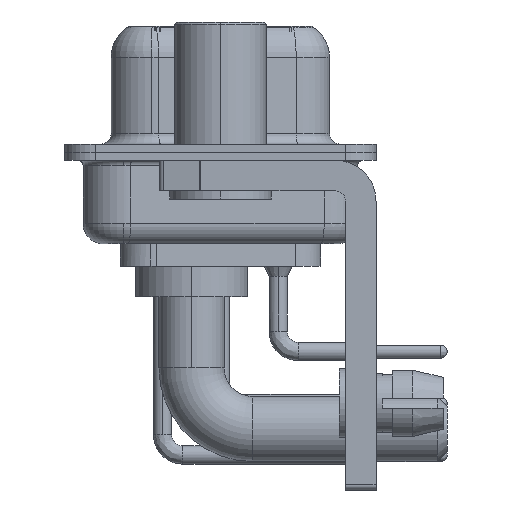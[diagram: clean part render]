
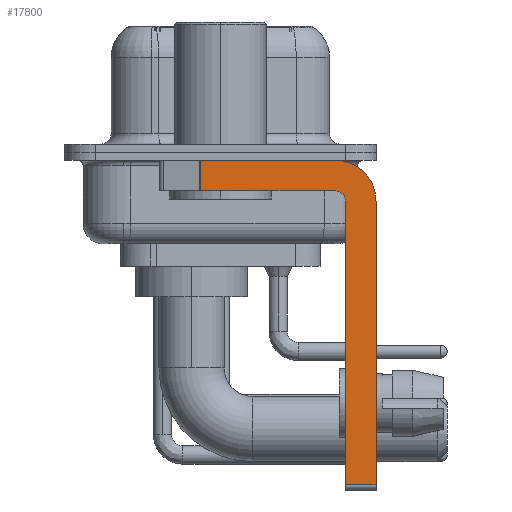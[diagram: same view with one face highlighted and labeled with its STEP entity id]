
A CAD part, left-side view. The second image highlights one B-rep face of the part: STEP entity #17800.
In plain terms, the highlighted planar face has unit normal (-1, 0, 0).
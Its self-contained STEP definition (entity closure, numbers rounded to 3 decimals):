
#389 = VERTEX_POINT ( 'NONE', #1475 ) ;
#677 = AXIS2_PLACEMENT_3D ( 'NONE', #33064, #6649, #15701 ) ;
#1475 = CARTESIAN_POINT ( 'NONE',  ( -2.9, 0.978, -1.9 ) ) ;
#1674 = LINE ( 'NONE', #5129, #32467 ) ;
#1938 = LINE ( 'NONE', #31788, #30900 ) ;
#2028 = LINE ( 'NONE', #25527, #17283 ) ;
#2201 = ORIENTED_EDGE ( 'NONE', *, *, #25031, .T. ) ;
#3866 = CARTESIAN_POINT ( 'NONE',  ( -2.9, -7.65, -2.4 ) ) ;
#3935 = AXIS2_PLACEMENT_3D ( 'NONE', #27962, #4063, #18531 ) ;
#4063 = DIRECTION ( 'NONE',  ( 1., 0., 0. ) ) ;
#4887 = VERTEX_POINT ( 'NONE', #8869 ) ;
#5129 = CARTESIAN_POINT ( 'NONE',  ( -2.9, 3., -0.4 ) ) ;
#5959 = LINE ( 'NONE', #26397, #6907 ) ;
#6649 = DIRECTION ( 'NONE',  ( -1., 0., 0. ) ) ;
#6763 = FACE_OUTER_BOUND ( 'NONE', #11766, .T. ) ;
#6823 = CIRCLE ( 'NONE', #677, 0.5 ) ;
#6907 = VECTOR ( 'NONE', #32362, 1000. ) ;
#7520 = PLANE ( 'NONE',  #3935 ) ;
#8081 = DIRECTION ( 'NONE',  ( 0., 0., 1. ) ) ;
#8353 = ORIENTED_EDGE ( 'NONE', *, *, #16531, .F. ) ;
#8869 = CARTESIAN_POINT ( 'NONE',  ( -2.9, -6.15, -16.35 ) ) ;
#9075 = VECTOR ( 'NONE', #13541, 1000. ) ;
#10257 = VERTEX_POINT ( 'NONE', #33871 ) ;
#10766 = VERTEX_POINT ( 'NONE', #16706 ) ;
#11649 = CIRCLE ( 'NONE', #35049, 2. ) ;
#11766 = EDGE_LOOP ( 'NONE', ( #28055, #37868, #34903, #28811, #8353, #2201, #26903, #27491 ) ) ;
#12780 = CARTESIAN_POINT ( 'NONE',  ( -2.9, -5.65, -16.35 ) ) ;
#13541 = DIRECTION ( 'NONE',  ( 0., -1., 0. ) ) ;
#13992 = CARTESIAN_POINT ( 'NONE',  ( -2.9, -5.65, -1.9 ) ) ;
#15282 = LINE ( 'NONE', #29932, #34259 ) ;
#15701 = DIRECTION ( 'NONE',  ( 0., 0., 1. ) ) ;
#16531 = EDGE_CURVE ( 'NONE', #4887, #10257, #1938, .T. ) ;
#16626 = EDGE_CURVE ( 'NONE', #31880, #10766, #5959, .T. ) ;
#16664 = DIRECTION ( 'NONE',  ( 0., 1., 0. ) ) ;
#16706 = CARTESIAN_POINT ( 'NONE',  ( -2.9, -7.65, -16.35 ) ) ;
#16936 = CARTESIAN_POINT ( 'NONE',  ( -2.9, 0.978, -0.4 ) ) ;
#17283 = VECTOR ( 'NONE', #16664, 1000. ) ;
#17800 = ADVANCED_FACE ( 'NONE', ( #6763 ), #7520, .F. ) ;
#18531 = DIRECTION ( 'NONE',  ( 0., 0., -1. ) ) ;
#18660 = DIRECTION ( 'NONE',  ( 1., 0., 0. ) ) ;
#18956 = LINE ( 'NONE', #12780, #9075 ) ;
#19241 = VERTEX_POINT ( 'NONE', #32858 ) ;
#21357 = DIRECTION ( 'NONE',  ( 0., 0., -1. ) ) ;
#24742 = DIRECTION ( 'NONE',  ( 0., 0., -1. ) ) ;
#25031 = EDGE_CURVE ( 'NONE', #4887, #10766, #18956, .T. ) ;
#25527 = CARTESIAN_POINT ( 'NONE',  ( -2.9, -5.65, -1.9 ) ) ;
#26397 = CARTESIAN_POINT ( 'NONE',  ( -2.9, -7.65, -2.4 ) ) ;
#26903 = ORIENTED_EDGE ( 'NONE', *, *, #16626, .F. ) ;
#27491 = ORIENTED_EDGE ( 'NONE', *, *, #37072, .F. ) ;
#27936 = EDGE_CURVE ( 'NONE', #10257, #32421, #6823, .T. ) ;
#27962 = CARTESIAN_POINT ( 'NONE',  ( -2.9, -5.65, -2.4 ) ) ;
#28055 = ORIENTED_EDGE ( 'NONE', *, *, #34947, .F. ) ;
#28811 = ORIENTED_EDGE ( 'NONE', *, *, #27936, .F. ) ;
#29322 = EDGE_CURVE ( 'NONE', #32421, #389, #2028, .T. ) ;
#29932 = CARTESIAN_POINT ( 'NONE',  ( -2.9, 0.978, -1.9 ) ) ;
#30900 = VECTOR ( 'NONE', #8081, 1000. ) ;
#31788 = CARTESIAN_POINT ( 'NONE',  ( -2.9, -6.15, -16.6 ) ) ;
#31880 = VERTEX_POINT ( 'NONE', #3866 ) ;
#32362 = DIRECTION ( 'NONE',  ( 0., 0., -1. ) ) ;
#32421 = VERTEX_POINT ( 'NONE', #13992 ) ;
#32467 = VECTOR ( 'NONE', #34622, 1000. ) ;
#32858 = CARTESIAN_POINT ( 'NONE',  ( -2.9, -5.65, -0.4 ) ) ;
#33064 = CARTESIAN_POINT ( 'NONE',  ( -2.9, -5.65, -2.4 ) ) ;
#33204 = EDGE_CURVE ( 'NONE', #35929, #389, #15282, .T. ) ;
#33871 = CARTESIAN_POINT ( 'NONE',  ( -2.9, -6.15, -2.4 ) ) ;
#34259 = VECTOR ( 'NONE', #24742, 1000. ) ;
#34622 = DIRECTION ( 'NONE',  ( 0., -1., 0. ) ) ;
#34903 = ORIENTED_EDGE ( 'NONE', *, *, #29322, .F. ) ;
#34947 = EDGE_CURVE ( 'NONE', #35929, #19241, #1674, .T. ) ;
#35049 = AXIS2_PLACEMENT_3D ( 'NONE', #36969, #18660, #21357 ) ;
#35929 = VERTEX_POINT ( 'NONE', #16936 ) ;
#36969 = CARTESIAN_POINT ( 'NONE',  ( -2.9, -5.65, -2.4 ) ) ;
#37072 = EDGE_CURVE ( 'NONE', #19241, #31880, #11649, .T. ) ;
#37868 = ORIENTED_EDGE ( 'NONE', *, *, #33204, .T. ) ;
